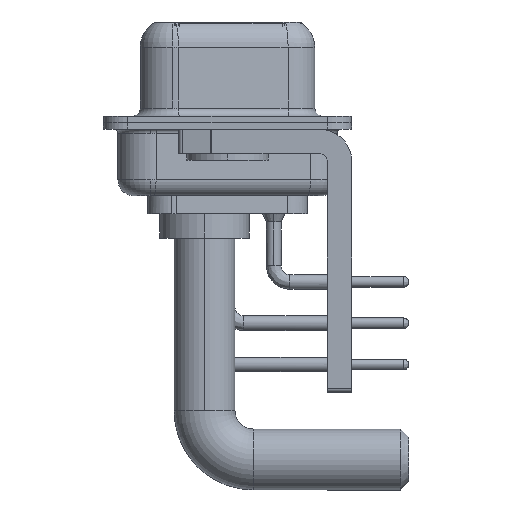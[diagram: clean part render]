
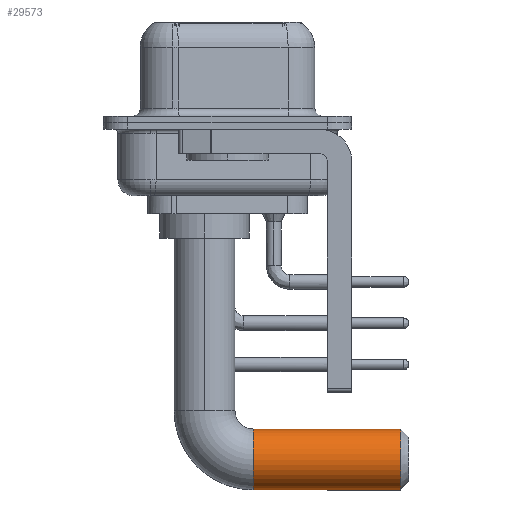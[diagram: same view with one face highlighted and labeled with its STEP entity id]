
A CAD part, left-side view. The second image highlights one B-rep face of the part: STEP entity #29573.
In plain terms, the highlighted cylindrical face has radius 1.875 mm (diameter 3.75 mm), a partial arc.
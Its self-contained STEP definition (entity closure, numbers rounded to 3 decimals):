
#675 = VERTEX_POINT ( 'NONE', #5531 ) ;
#924 = CIRCLE ( 'NONE', #16500, 1.875 ) ;
#1154 = CARTESIAN_POINT ( 'NONE',  ( 0., -3., -15.505 ) ) ;
#1275 = ORIENTED_EDGE ( 'NONE', *, *, #8372, .F. ) ;
#1353 = CARTESIAN_POINT ( 'NONE',  ( 0., -3., -15.505 ) ) ;
#3686 = CARTESIAN_POINT ( 'NONE',  ( 0., -12.07, -13.63 ) ) ;
#3777 = CARTESIAN_POINT ( 'NONE',  ( 0., -12.07, -15.505 ) ) ;
#3941 = ORIENTED_EDGE ( 'NONE', *, *, #27151, .T. ) ;
#5531 = CARTESIAN_POINT ( 'NONE',  ( 0., -12.07, -11.755 ) ) ;
#5917 = LINE ( 'NONE', #1353, #22966 ) ;
#6653 = CYLINDRICAL_SURFACE ( 'NONE', #19178, 1.875 ) ;
#7115 = CARTESIAN_POINT ( 'NONE',  ( 0., -3., -13.63 ) ) ;
#8372 = EDGE_CURVE ( 'NONE', #27898, #675, #19107, .T. ) ;
#9102 = DIRECTION ( 'NONE',  ( 0., -1., 0. ) ) ;
#9433 = CARTESIAN_POINT ( 'NONE',  ( 0., -3., -11.755 ) ) ;
#10890 = ORIENTED_EDGE ( 'NONE', *, *, #20046, .T. ) ;
#11683 = VERTEX_POINT ( 'NONE', #1154 ) ;
#14106 = DIRECTION ( 'NONE',  ( -1., 0., 0. ) ) ;
#16139 = VERTEX_POINT ( 'NONE', #3777 ) ;
#16249 = FACE_OUTER_BOUND ( 'NONE', #22899, .T. ) ;
#16413 = DIRECTION ( 'NONE',  ( 0., -1., 0. ) ) ;
#16450 = EDGE_CURVE ( 'NONE', #27898, #11683, #28091, .T. ) ;
#16500 = AXIS2_PLACEMENT_3D ( 'NONE', #3686, #24389, #24698 ) ;
#19107 = LINE ( 'NONE', #28391, #23831 ) ;
#19178 = AXIS2_PLACEMENT_3D ( 'NONE', #25532, #9102, #25223 ) ;
#20046 = EDGE_CURVE ( 'NONE', #11683, #16139, #5917, .T. ) ;
#21183 = ORIENTED_EDGE ( 'NONE', *, *, #16450, .T. ) ;
#21625 = DIRECTION ( 'NONE',  ( 0., -1., 0. ) ) ;
#22899 = EDGE_LOOP ( 'NONE', ( #1275, #21183, #10890, #3941 ) ) ;
#22966 = VECTOR ( 'NONE', #21625, 1000. ) ;
#23831 = VECTOR ( 'NONE', #27403, 1000. ) ;
#24389 = DIRECTION ( 'NONE',  ( 0., 1., 0. ) ) ;
#24698 = DIRECTION ( 'NONE',  ( 0., 0., -1. ) ) ;
#25223 = DIRECTION ( 'NONE',  ( 0., 0., -1. ) ) ;
#25532 = CARTESIAN_POINT ( 'NONE',  ( 0., -3., -13.63 ) ) ;
#27151 = EDGE_CURVE ( 'NONE', #16139, #675, #924, .T. ) ;
#27403 = DIRECTION ( 'NONE',  ( 0., -1., 0. ) ) ;
#27601 = AXIS2_PLACEMENT_3D ( 'NONE', #7115, #16413, #14106 ) ;
#27898 = VERTEX_POINT ( 'NONE', #9433 ) ;
#28091 = CIRCLE ( 'NONE', #27601, 1.875 ) ;
#28391 = CARTESIAN_POINT ( 'NONE',  ( 0., -3., -11.755 ) ) ;
#29573 = ADVANCED_FACE ( 'NONE', ( #16249 ), #6653, .T. ) ;
